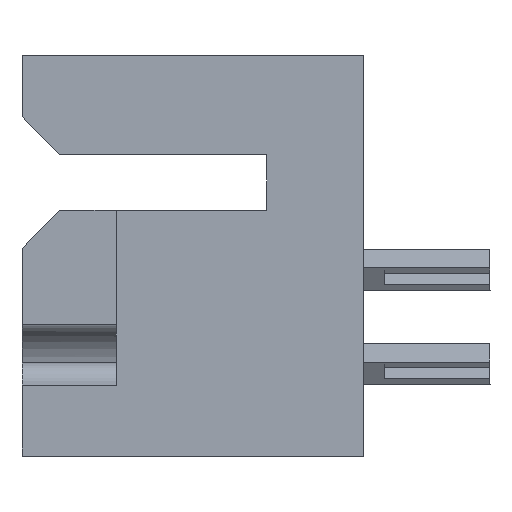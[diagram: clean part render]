
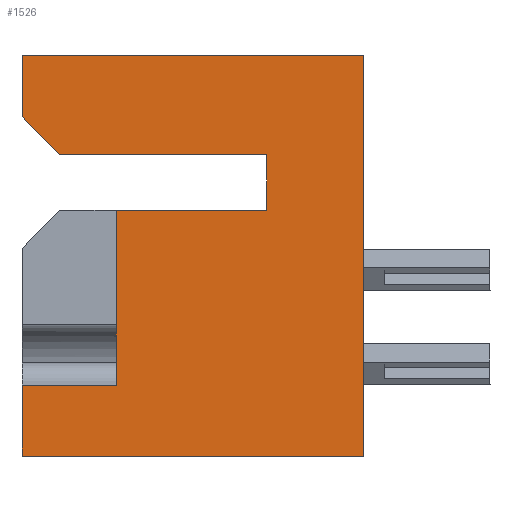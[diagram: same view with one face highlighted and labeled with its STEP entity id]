
A CAD part, left-side view. The second image highlights one B-rep face of the part: STEP entity #1526.
In plain terms, the highlighted planar face has unit normal (-1, 0, 0).
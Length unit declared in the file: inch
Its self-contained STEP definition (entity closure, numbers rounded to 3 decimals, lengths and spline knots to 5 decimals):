
#35 = CARTESIAN_POINT ( 'NONE',  ( 0., 0.453, 0. ) ) ;
#275 = VECTOR ( 'NONE', #1611, 39.37008 ) ;
#585 = EDGE_CURVE ( 'NONE', #14736, #21643, #13791, .T. ) ;
#935 = LINE ( 'NONE', #11731, #9479 ) ;
#1209 = VECTOR ( 'NONE', #11780, 39.37008 ) ;
#1240 = CARTESIAN_POINT ( 'NONE',  ( 0., 0.453, -0.531 ) ) ;
#1526 = ADVANCED_FACE ( 'NONE', ( #17037 ), #7176, .F. ) ;
#1611 = DIRECTION ( 'NONE',  ( 0., 0., 1. ) ) ;
#1815 = ORIENTED_EDGE ( 'NONE', *, *, #22445, .F. ) ;
#2081 = CARTESIAN_POINT ( 'NONE',  ( 0., 0.453, -0.081 ) ) ;
#2279 = CARTESIAN_POINT ( 'NONE',  ( 0., 0.403, -0.131 ) ) ;
#2497 = ORIENTED_EDGE ( 'NONE', *, *, #4084, .F. ) ;
#2922 = VERTEX_POINT ( 'NONE', #24233 ) ;
#3121 = VERTEX_POINT ( 'NONE', #14423 ) ;
#3170 = ORIENTED_EDGE ( 'NONE', *, *, #14773, .F. ) ;
#3385 = DIRECTION ( 'NONE',  ( 0., 0., 1. ) ) ;
#3896 = CARTESIAN_POINT ( 'NONE',  ( 0., 0.453, 0. ) ) ;
#3948 = ORIENTED_EDGE ( 'NONE', *, *, #15141, .F. ) ;
#4084 = EDGE_CURVE ( 'NONE', #14736, #24029, #19224, .T. ) ;
#4178 = CARTESIAN_POINT ( 'NONE',  ( 0., 0.328, -0.437 ) ) ;
#4368 = VECTOR ( 'NONE', #22857, 39.37008 ) ;
#4431 = CARTESIAN_POINT ( 'NONE',  ( 0., 0.128, -0.131 ) ) ;
#4671 = ORIENTED_EDGE ( 'NONE', *, *, #5108, .T. ) ;
#4818 = CARTESIAN_POINT ( 'NONE',  ( 0., 0.128, -0.205 ) ) ;
#5108 = EDGE_CURVE ( 'NONE', #20010, #19506, #22422, .T. ) ;
#5576 = LINE ( 'NONE', #1240, #22334 ) ;
#6106 = VERTEX_POINT ( 'NONE', #9675 ) ;
#7176 = PLANE ( 'NONE',  #25330 ) ;
#7297 = VERTEX_POINT ( 'NONE', #24849 ) ;
#7367 = DIRECTION ( 'NONE',  ( 1., 0., 0. ) ) ;
#8356 = ORIENTED_EDGE ( 'NONE', *, *, #22891, .T. ) ;
#8939 = ORIENTED_EDGE ( 'NONE', *, *, #23863, .T. ) ;
#9255 = CARTESIAN_POINT ( 'NONE',  ( 0., 0.453, 0. ) ) ;
#9479 = VECTOR ( 'NONE', #3385, 39.37008 ) ;
#9675 = CARTESIAN_POINT ( 'NONE',  ( 0., 0., -0.531 ) ) ;
#10169 = ORIENTED_EDGE ( 'NONE', *, *, #13798, .F. ) ;
#10352 = CARTESIAN_POINT ( 'NONE',  ( 0., 0.453, -0.437 ) ) ;
#10383 = CARTESIAN_POINT ( 'NONE',  ( 0., 0.328, -0.437 ) ) ;
#10597 = CARTESIAN_POINT ( 'NONE',  ( 0., 0.328, -0.205 ) ) ;
#11731 = CARTESIAN_POINT ( 'NONE',  ( 0., 0.128, -0.131 ) ) ;
#11780 = DIRECTION ( 'NONE',  ( 0., 1., 0. ) ) ;
#12318 = CARTESIAN_POINT ( 'NONE',  ( 0., 0.403, -0.131 ) ) ;
#12513 = DIRECTION ( 'NONE',  ( 0., 1., 0. ) ) ;
#13118 = VECTOR ( 'NONE', #12513, 39.37008 ) ;
#13261 = LINE ( 'NONE', #4818, #20203 ) ;
#13758 = EDGE_CURVE ( 'NONE', #2922, #6106, #5576, .T. ) ;
#13791 = LINE ( 'NONE', #10383, #13118 ) ;
#13798 = EDGE_CURVE ( 'NONE', #2922, #21643, #27224, .T. ) ;
#14082 = VECTOR ( 'NONE', #16704, 39.37008 ) ;
#14208 = CARTESIAN_POINT ( 'NONE',  ( 0., 0.128, -0.131 ) ) ;
#14242 = ORIENTED_EDGE ( 'NONE', *, *, #585, .T. ) ;
#14261 = DIRECTION ( 'NONE',  ( 0., 0., 1. ) ) ;
#14418 = EDGE_CURVE ( 'NONE', #3121, #26522, #935, .T. ) ;
#14423 = CARTESIAN_POINT ( 'NONE',  ( 0., 0.128, -0.205 ) ) ;
#14736 = VERTEX_POINT ( 'NONE', #4178 ) ;
#14773 = EDGE_CURVE ( 'NONE', #7297, #18905, #22594, .T. ) ;
#15141 = EDGE_CURVE ( 'NONE', #26522, #19506, #25195, .T. ) ;
#15179 = ORIENTED_EDGE ( 'NONE', *, *, #13758, .T. ) ;
#15635 = VECTOR ( 'NONE', #14261, 39.37008 ) ;
#16390 = CARTESIAN_POINT ( 'NONE',  ( 0., 0.328, -0.205 ) ) ;
#16704 = DIRECTION ( 'NONE',  ( 0., -1., 0. ) ) ;
#17037 = FACE_OUTER_BOUND ( 'NONE', #26774, .T. ) ;
#18140 = CARTESIAN_POINT ( 'NONE',  ( 0., 0., 0. ) ) ;
#18184 = DIRECTION ( 'NONE',  ( 0., 1., 0. ) ) ;
#18348 = DIRECTION ( 'NONE',  ( 0., -0.707, -0.707 ) ) ;
#18905 = VERTEX_POINT ( 'NONE', #25865 ) ;
#18983 = DIRECTION ( 'NONE',  ( 0., 0., 1. ) ) ;
#19224 = LINE ( 'NONE', #10597, #4368 ) ;
#19506 = VERTEX_POINT ( 'NONE', #2279 ) ;
#20010 = VERTEX_POINT ( 'NONE', #2081 ) ;
#20203 = VECTOR ( 'NONE', #18184, 39.37008 ) ;
#21643 = VERTEX_POINT ( 'NONE', #10352 ) ;
#22334 = VECTOR ( 'NONE', #24299, 39.37008 ) ;
#22422 = LINE ( 'NONE', #12318, #24704 ) ;
#22445 = EDGE_CURVE ( 'NONE', #20010, #7297, #23187, .T. ) ;
#22594 = LINE ( 'NONE', #35, #14082 ) ;
#22857 = DIRECTION ( 'NONE',  ( 0., 0., 1. ) ) ;
#22891 = EDGE_CURVE ( 'NONE', #6106, #18905, #23515, .T. ) ;
#23187 = LINE ( 'NONE', #25087, #24169 ) ;
#23515 = LINE ( 'NONE', #18140, #15635 ) ;
#23863 = EDGE_CURVE ( 'NONE', #3121, #24029, #13261, .T. ) ;
#23964 = DIRECTION ( 'NONE',  ( 0., 0., -1. ) ) ;
#24029 = VERTEX_POINT ( 'NONE', #16390 ) ;
#24169 = VECTOR ( 'NONE', #18983, 39.37008 ) ;
#24233 = CARTESIAN_POINT ( 'NONE',  ( 0., 0.453, -0.531 ) ) ;
#24299 = DIRECTION ( 'NONE',  ( 0., -1., 0. ) ) ;
#24704 = VECTOR ( 'NONE', #18348, 39.37008 ) ;
#24849 = CARTESIAN_POINT ( 'NONE',  ( 0., 0.453, 0. ) ) ;
#25087 = CARTESIAN_POINT ( 'NONE',  ( 0., 0.453, 0. ) ) ;
#25195 = LINE ( 'NONE', #14208, #1209 ) ;
#25330 = AXIS2_PLACEMENT_3D ( 'NONE', #9255, #7367, #23964 ) ;
#25865 = CARTESIAN_POINT ( 'NONE',  ( 0., 0., 0. ) ) ;
#26522 = VERTEX_POINT ( 'NONE', #4431 ) ;
#26605 = ORIENTED_EDGE ( 'NONE', *, *, #14418, .F. ) ;
#26774 = EDGE_LOOP ( 'NONE', ( #14242, #10169, #15179, #8356, #3170, #1815, #4671, #3948, #26605, #8939, #2497 ) ) ;
#27224 = LINE ( 'NONE', #3896, #275 ) ;
